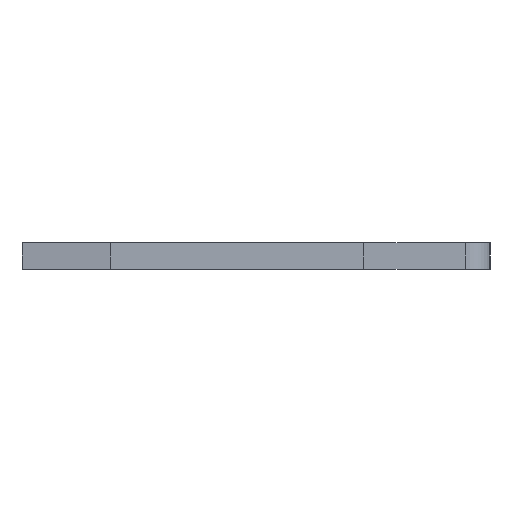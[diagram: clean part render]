
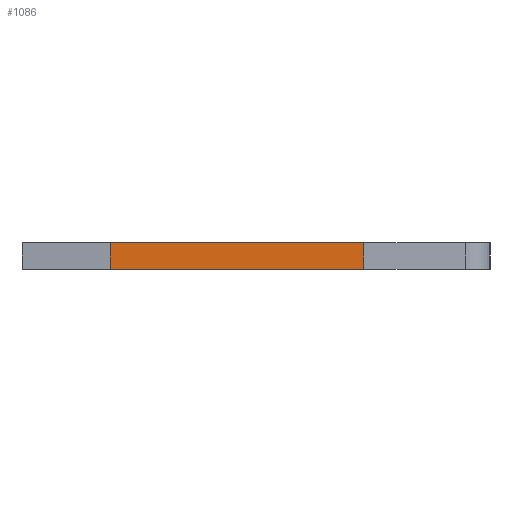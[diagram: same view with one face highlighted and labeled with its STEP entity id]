
A CAD part, left-side view. The second image highlights one B-rep face of the part: STEP entity #1086.
In plain terms, the highlighted face is planar.
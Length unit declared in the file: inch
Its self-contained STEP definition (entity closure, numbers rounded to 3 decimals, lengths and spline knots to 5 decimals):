
#90 = EDGE_LOOP ( 'NONE', ( #576, #145, #1430, #546 ) ) ;
#120 = CARTESIAN_POINT ( 'NONE',  ( 0.013, 0.146, -0.0575 ) ) ;
#145 = ORIENTED_EDGE ( 'NONE', *, *, #534, .F. ) ;
#150 = CARTESIAN_POINT ( 'NONE',  ( 0.013, 0.146, -0.0575 ) ) ;
#157 = DIRECTION ( 'NONE',  ( -1., 0., 0. ) ) ;
#204 = LINE ( 'NONE', #1375, #1333 ) ;
#215 = CARTESIAN_POINT ( 'NONE',  ( -0.013, -0.099, -0.0575 ) ) ;
#427 = CARTESIAN_POINT ( 'NONE',  ( 0.013, 0.146, -0.0575 ) ) ;
#463 = AXIS2_PLACEMENT_3D ( 'NONE', #427, #1237, #1346 ) ;
#534 = EDGE_CURVE ( 'NONE', #1217, #732, #673, .T. ) ;
#546 = ORIENTED_EDGE ( 'NONE', *, *, #771, .T. ) ;
#570 = FACE_OUTER_BOUND ( 'NONE', #90, .T. ) ;
#576 = ORIENTED_EDGE ( 'NONE', *, *, #1321, .T. ) ;
#589 = CARTESIAN_POINT ( 'NONE',  ( 0.013, 0.146, -0.0575 ) ) ;
#624 = DIRECTION ( 'NONE',  ( -1., 0., 0. ) ) ;
#640 = EDGE_CURVE ( 'NONE', #1040, #1217, #692, .T. ) ;
#673 = LINE ( 'NONE', #589, #1125 ) ;
#692 = LINE ( 'NONE', #150, #1109 ) ;
#732 = VERTEX_POINT ( 'NONE', #822 ) ;
#771 = EDGE_CURVE ( 'NONE', #1040, #1016, #1228, .T. ) ;
#801 = DIRECTION ( 'NONE',  ( 0., 1., 0. ) ) ;
#822 = CARTESIAN_POINT ( 'NONE',  ( -0.013, 0.146, -0.0575 ) ) ;
#997 = CARTESIAN_POINT ( 'NONE',  ( 0.013, -0.099, -0.0575 ) ) ;
#1016 = VERTEX_POINT ( 'NONE', #215 ) ;
#1040 = VERTEX_POINT ( 'NONE', #997 ) ;
#1086 = ADVANCED_FACE ( 'NONE', ( #570 ), #1101, .F. ) ;
#1101 = PLANE ( 'NONE',  #463 ) ;
#1109 = VECTOR ( 'NONE', #1400, 39.37008 ) ;
#1125 = VECTOR ( 'NONE', #157, 39.37008 ) ;
#1217 = VERTEX_POINT ( 'NONE', #120 ) ;
#1228 = LINE ( 'NONE', #1442, #1243 ) ;
#1237 = DIRECTION ( 'NONE',  ( 0., 0., 1. ) ) ;
#1243 = VECTOR ( 'NONE', #624, 39.37008 ) ;
#1321 = EDGE_CURVE ( 'NONE', #1016, #732, #204, .T. ) ;
#1333 = VECTOR ( 'NONE', #801, 39.37008 ) ;
#1346 = DIRECTION ( 'NONE',  ( 1., 0., 0. ) ) ;
#1375 = CARTESIAN_POINT ( 'NONE',  ( -0.013, 0.146, -0.0575 ) ) ;
#1400 = DIRECTION ( 'NONE',  ( 0., 1., 0. ) ) ;
#1430 = ORIENTED_EDGE ( 'NONE', *, *, #640, .F. ) ;
#1442 = CARTESIAN_POINT ( 'NONE',  ( 0.013, -0.099, -0.0575 ) ) ;
